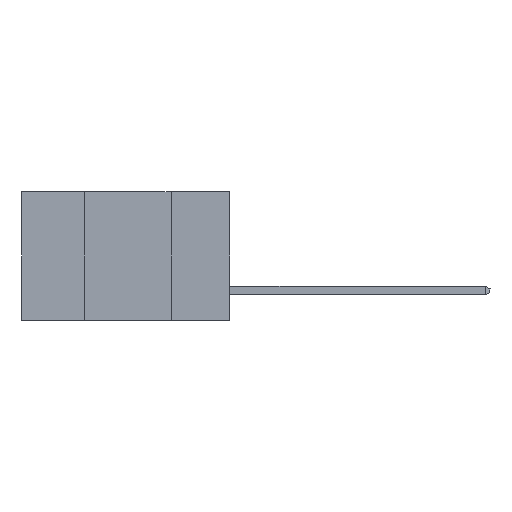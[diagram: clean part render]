
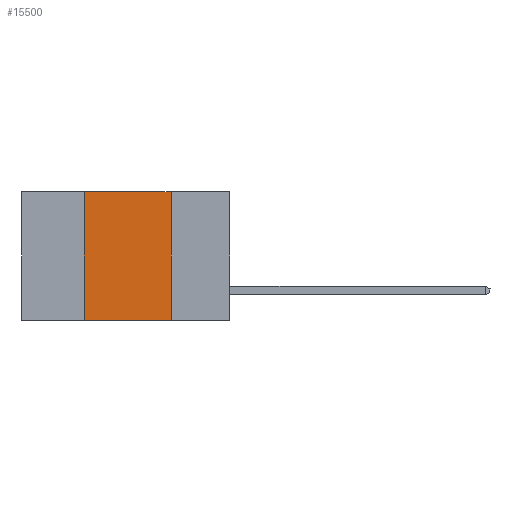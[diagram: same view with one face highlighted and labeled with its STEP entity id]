
A CAD part, left-side view. The second image highlights one B-rep face of the part: STEP entity #15500.
In plain terms, the highlighted planar face has unit normal (-1, 0, 0).
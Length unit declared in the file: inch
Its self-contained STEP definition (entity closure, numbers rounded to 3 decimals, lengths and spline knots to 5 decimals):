
#433 = VECTOR ( 'NONE', #6427, 39.37008 ) ;
#1547 = CARTESIAN_POINT ( 'NONE',  ( 0., 0.42, 0. ) ) ;
#1848 = DIRECTION ( 'NONE',  ( 0., 0., -1. ) ) ;
#2160 = VERTEX_POINT ( 'NONE', #10034 ) ;
#2418 = VECTOR ( 'NONE', #4182, 39.37008 ) ;
#2600 = LINE ( 'NONE', #9030, #433 ) ;
#4182 = DIRECTION ( 'NONE',  ( 0., -1., 0. ) ) ;
#4441 = PLANE ( 'NONE',  #12931 ) ;
#4904 = CARTESIAN_POINT ( 'NONE',  ( 0., 0.42, 0. ) ) ;
#4937 = ORIENTED_EDGE ( 'NONE', *, *, #6995, .F. ) ;
#5364 = CARTESIAN_POINT ( 'NONE',  ( 0., 0.6, 0. ) ) ;
#5617 = DIRECTION ( 'NONE',  ( 1., 0., 0. ) ) ;
#5664 = ORIENTED_EDGE ( 'NONE', *, *, #14248, .F. ) ;
#5807 = CARTESIAN_POINT ( 'NONE',  ( 0., 0.17, 0. ) ) ;
#6427 = DIRECTION ( 'NONE',  ( 0., 0., -1. ) ) ;
#6854 = VERTEX_POINT ( 'NONE', #8558 ) ;
#6887 = ORIENTED_EDGE ( 'NONE', *, *, #16057, .F. ) ;
#6892 = LINE ( 'NONE', #15376, #12862 ) ;
#6995 = EDGE_CURVE ( 'NONE', #10381, #2160, #2600, .T. ) ;
#8482 = LINE ( 'NONE', #1547, #15624 ) ;
#8558 = CARTESIAN_POINT ( 'NONE',  ( 0., 0.42, -0.37 ) ) ;
#9030 = CARTESIAN_POINT ( 'NONE',  ( 0., 0.17, 0. ) ) ;
#10034 = CARTESIAN_POINT ( 'NONE',  ( 0., 0.17, -0.37 ) ) ;
#10381 = VERTEX_POINT ( 'NONE', #5807 ) ;
#10541 = DIRECTION ( 'NONE',  ( 0., 0., 1. ) ) ;
#10753 = ORIENTED_EDGE ( 'NONE', *, *, #15781, .T. ) ;
#12201 = EDGE_LOOP ( 'NONE', ( #4937, #5664, #6887, #10753 ) ) ;
#12697 = VERTEX_POINT ( 'NONE', #4904 ) ;
#12862 = VECTOR ( 'NONE', #13190, 39.37008 ) ;
#12931 = AXIS2_PLACEMENT_3D ( 'NONE', #14488, #5617, #1848 ) ;
#13190 = DIRECTION ( 'NONE',  ( 0., -1., 0. ) ) ;
#14248 = EDGE_CURVE ( 'NONE', #12697, #10381, #15116, .T. ) ;
#14488 = CARTESIAN_POINT ( 'NONE',  ( 0., 0.6, 0. ) ) ;
#15067 = FACE_OUTER_BOUND ( 'NONE', #12201, .T. ) ;
#15116 = LINE ( 'NONE', #5364, #2418 ) ;
#15376 = CARTESIAN_POINT ( 'NONE',  ( 0., 0.6, -0.37 ) ) ;
#15500 = ADVANCED_FACE ( 'NONE', ( #15067 ), #4441, .F. ) ;
#15624 = VECTOR ( 'NONE', #10541, 39.37008 ) ;
#15781 = EDGE_CURVE ( 'NONE', #6854, #2160, #6892, .T. ) ;
#16057 = EDGE_CURVE ( 'NONE', #6854, #12697, #8482, .T. ) ;
